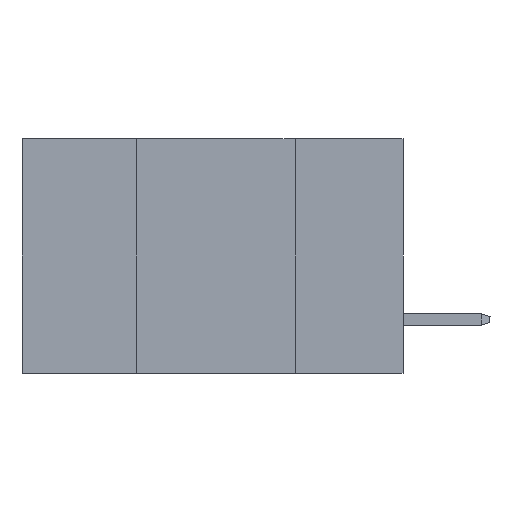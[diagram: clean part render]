
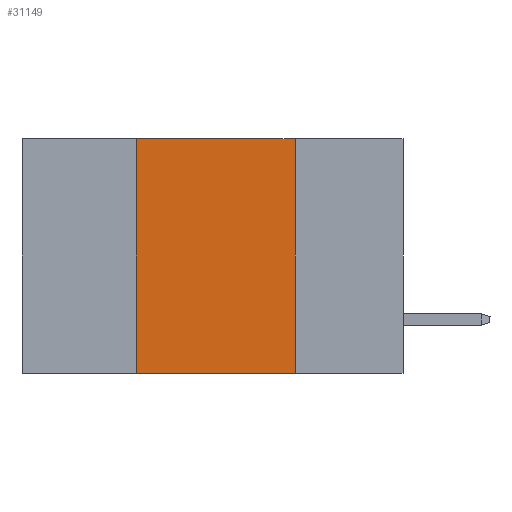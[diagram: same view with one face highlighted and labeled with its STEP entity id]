
A CAD part, left-side view. The second image highlights one B-rep face of the part: STEP entity #31149.
In plain terms, the highlighted planar face has unit normal (-1, 0, 0).
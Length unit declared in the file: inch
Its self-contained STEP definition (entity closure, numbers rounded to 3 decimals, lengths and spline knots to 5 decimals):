
#1164 = DIRECTION ( 'NONE',  ( 0., 0., 1. ) ) ;
#1428 = CARTESIAN_POINT ( 'NONE',  ( 0., 0.17, -0.37 ) ) ;
#1487 = VECTOR ( 'NONE', #27659, 39.37008 ) ;
#2260 = ORIENTED_EDGE ( 'NONE', *, *, #14168, .F. ) ;
#3124 = VECTOR ( 'NONE', #12692, 39.37008 ) ;
#3188 = AXIS2_PLACEMENT_3D ( 'NONE', #4804, #22367, #7719 ) ;
#3212 = ORIENTED_EDGE ( 'NONE', *, *, #14758, .F. ) ;
#3289 = ORIENTED_EDGE ( 'NONE', *, *, #11637, .F. ) ;
#3481 = LINE ( 'NONE', #31257, #1487 ) ;
#4070 = LINE ( 'NONE', #13601, #20670 ) ;
#4804 = CARTESIAN_POINT ( 'NONE',  ( 0., 0.6, 0. ) ) ;
#4983 = VERTEX_POINT ( 'NONE', #30378 ) ;
#6269 = VERTEX_POINT ( 'NONE', #15249 ) ;
#6751 = CARTESIAN_POINT ( 'NONE',  ( 0., 0.6, -0.37 ) ) ;
#7089 = VERTEX_POINT ( 'NONE', #1428 ) ;
#7380 = CARTESIAN_POINT ( 'NONE',  ( 0., 0.42, 0. ) ) ;
#7719 = DIRECTION ( 'NONE',  ( 0., 0., -1. ) ) ;
#11637 = EDGE_CURVE ( 'NONE', #13621, #4983, #3481, .T. ) ;
#12692 = DIRECTION ( 'NONE',  ( 0., 0., -1. ) ) ;
#13601 = CARTESIAN_POINT ( 'NONE',  ( 0., 0.42, 0. ) ) ;
#13621 = VERTEX_POINT ( 'NONE', #7380 ) ;
#14168 = EDGE_CURVE ( 'NONE', #6269, #13621, #4070, .T. ) ;
#14758 = EDGE_CURVE ( 'NONE', #4983, #7089, #28140, .T. ) ;
#15118 = CARTESIAN_POINT ( 'NONE',  ( 0., 0.17, 0. ) ) ;
#15249 = CARTESIAN_POINT ( 'NONE',  ( 0., 0.42, -0.37 ) ) ;
#16613 = DIRECTION ( 'NONE',  ( 0., -1., 0. ) ) ;
#16936 = FACE_OUTER_BOUND ( 'NONE', #28602, .T. ) ;
#20670 = VECTOR ( 'NONE', #1164, 39.37008 ) ;
#22367 = DIRECTION ( 'NONE',  ( 1., 0., 0. ) ) ;
#24075 = ORIENTED_EDGE ( 'NONE', *, *, #28144, .T. ) ;
#27659 = DIRECTION ( 'NONE',  ( 0., -1., 0. ) ) ;
#28140 = LINE ( 'NONE', #15118, #3124 ) ;
#28144 = EDGE_CURVE ( 'NONE', #6269, #7089, #28811, .T. ) ;
#28159 = VECTOR ( 'NONE', #16613, 39.37008 ) ;
#28602 = EDGE_LOOP ( 'NONE', ( #3212, #3289, #2260, #24075 ) ) ;
#28811 = LINE ( 'NONE', #6751, #28159 ) ;
#29593 = PLANE ( 'NONE',  #3188 ) ;
#30378 = CARTESIAN_POINT ( 'NONE',  ( 0., 0.17, 0. ) ) ;
#31149 = ADVANCED_FACE ( 'NONE', ( #16936 ), #29593, .F. ) ;
#31257 = CARTESIAN_POINT ( 'NONE',  ( 0., 0.6, 0. ) ) ;
